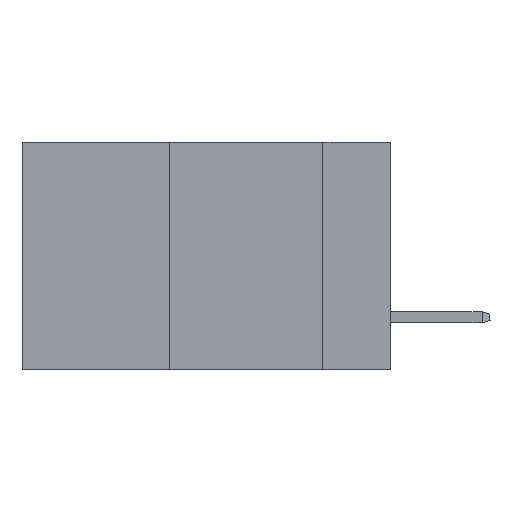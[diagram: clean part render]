
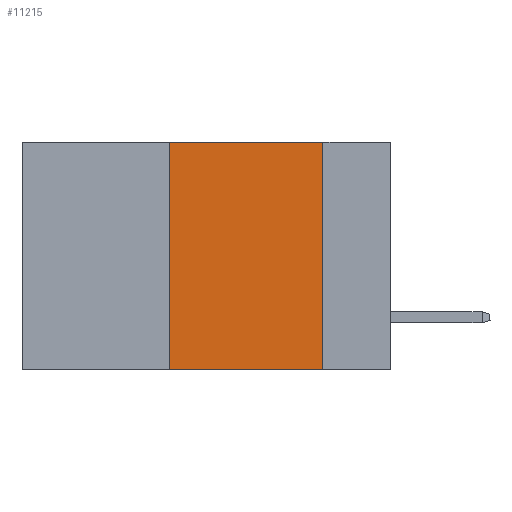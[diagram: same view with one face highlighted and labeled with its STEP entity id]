
A CAD part, left-side view. The second image highlights one B-rep face of the part: STEP entity #11215.
In plain terms, the highlighted planar face has unit normal (-1, 0, 0).
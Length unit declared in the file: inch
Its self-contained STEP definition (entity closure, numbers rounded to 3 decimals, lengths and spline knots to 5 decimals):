
#249 = CARTESIAN_POINT ( 'NONE',  ( 0., 0.36, -0.37 ) ) ;
#1262 = CARTESIAN_POINT ( 'NONE',  ( 0., 0.6, 0. ) ) ;
#1364 = CARTESIAN_POINT ( 'NONE',  ( 0., 0.11, -0.37 ) ) ;
#1398 = VERTEX_POINT ( 'NONE', #15169 ) ;
#2296 = PLANE ( 'NONE',  #10179 ) ;
#2409 = FACE_OUTER_BOUND ( 'NONE', #8513, .T. ) ;
#2507 = EDGE_CURVE ( 'NONE', #9783, #11321, #3430, .T. ) ;
#2685 = CARTESIAN_POINT ( 'NONE',  ( 0., 0.6, 0. ) ) ;
#2991 = VECTOR ( 'NONE', #5060, 39.37008 ) ;
#3430 = LINE ( 'NONE', #8991, #6459 ) ;
#4217 = VECTOR ( 'NONE', #15374, 39.37008 ) ;
#4359 = EDGE_CURVE ( 'NONE', #9783, #13208, #4588, .T. ) ;
#4588 = LINE ( 'NONE', #12963, #4217 ) ;
#4910 = ORIENTED_EDGE ( 'NONE', *, *, #2507, .T. ) ;
#5060 = DIRECTION ( 'NONE',  ( 0., -1., 0. ) ) ;
#5439 = CARTESIAN_POINT ( 'NONE',  ( 0., 0.36, 0. ) ) ;
#5797 = ORIENTED_EDGE ( 'NONE', *, *, #11783, .F. ) ;
#6084 = CARTESIAN_POINT ( 'NONE',  ( 0., 0.11, 0. ) ) ;
#6247 = DIRECTION ( 'NONE',  ( 0., 0., -1. ) ) ;
#6459 = VECTOR ( 'NONE', #7679, 39.37008 ) ;
#7363 = EDGE_CURVE ( 'NONE', #13208, #1398, #14150, .T. ) ;
#7600 = DIRECTION ( 'NONE',  ( 0., 0., -1. ) ) ;
#7679 = DIRECTION ( 'NONE',  ( 0., -1., 0. ) ) ;
#7745 = ORIENTED_EDGE ( 'NONE', *, *, #7363, .F. ) ;
#8513 = EDGE_LOOP ( 'NONE', ( #5797, #7745, #15609, #4910 ) ) ;
#8991 = CARTESIAN_POINT ( 'NONE',  ( 0., 0.6, -0.37 ) ) ;
#9620 = LINE ( 'NONE', #6084, #10560 ) ;
#9783 = VERTEX_POINT ( 'NONE', #249 ) ;
#10179 = AXIS2_PLACEMENT_3D ( 'NONE', #1262, #13587, #7600 ) ;
#10560 = VECTOR ( 'NONE', #6247, 39.37008 ) ;
#11215 = ADVANCED_FACE ( 'NONE', ( #2409 ), #2296, .F. ) ;
#11321 = VERTEX_POINT ( 'NONE', #1364 ) ;
#11783 = EDGE_CURVE ( 'NONE', #1398, #11321, #9620, .T. ) ;
#12963 = CARTESIAN_POINT ( 'NONE',  ( 0., 0.36, 0. ) ) ;
#13208 = VERTEX_POINT ( 'NONE', #5439 ) ;
#13587 = DIRECTION ( 'NONE',  ( 1., 0., 0. ) ) ;
#14150 = LINE ( 'NONE', #2685, #2991 ) ;
#15169 = CARTESIAN_POINT ( 'NONE',  ( 0., 0.11, 0. ) ) ;
#15374 = DIRECTION ( 'NONE',  ( 0., 0., 1. ) ) ;
#15609 = ORIENTED_EDGE ( 'NONE', *, *, #4359, .F. ) ;
